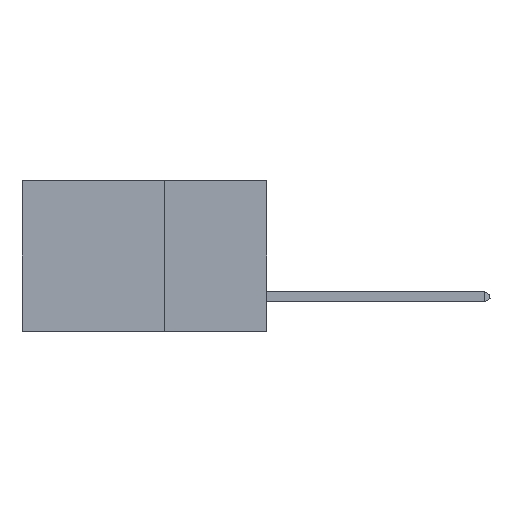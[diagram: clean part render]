
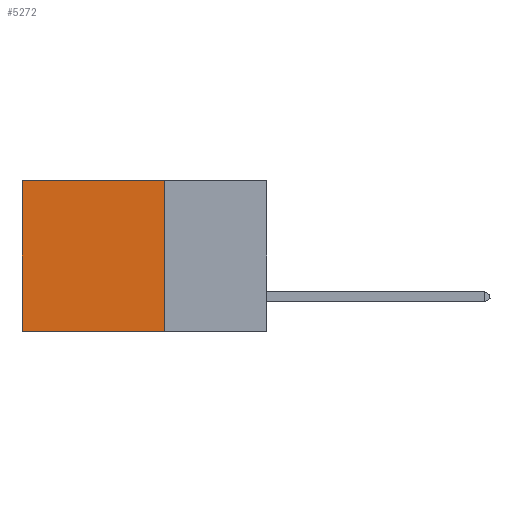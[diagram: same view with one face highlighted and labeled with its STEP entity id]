
A CAD part, left-side view. The second image highlights one B-rep face of the part: STEP entity #5272.
In plain terms, the highlighted planar face has unit normal (-1, 0, 0).
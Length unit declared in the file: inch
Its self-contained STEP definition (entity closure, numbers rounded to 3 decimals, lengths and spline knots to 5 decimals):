
#1403 = CARTESIAN_POINT ( 'NONE',  ( 0.2875, 0.25, -0.37 ) ) ;
#1807 = ORIENTED_EDGE ( 'NONE', *, *, #14989, .T. ) ;
#1818 = VERTEX_POINT ( 'NONE', #23253 ) ;
#1968 = LINE ( 'NONE', #18146, #23484 ) ;
#2635 = DIRECTION ( 'NONE',  ( 0., 0., -1. ) ) ;
#5272 = ADVANCED_FACE ( 'NONE', ( #17365 ), #20144, .F. ) ;
#7368 = CARTESIAN_POINT ( 'NONE',  ( 0.2875, 0.25, -0.37 ) ) ;
#7627 = DIRECTION ( 'NONE',  ( 0., 0., -1. ) ) ;
#8122 = CARTESIAN_POINT ( 'NONE',  ( 0.2875, 0.25, 0. ) ) ;
#8466 = EDGE_LOOP ( 'NONE', ( #1807, #14694, #33051, #15917 ) ) ;
#9896 = CARTESIAN_POINT ( 'NONE',  ( 0.2875, 0.25, 0. ) ) ;
#10427 = LINE ( 'NONE', #16208, #32858 ) ;
#11057 = VERTEX_POINT ( 'NONE', #1403 ) ;
#12004 = DIRECTION ( 'NONE',  ( 0., 1., 0. ) ) ;
#14694 = ORIENTED_EDGE ( 'NONE', *, *, #29916, .F. ) ;
#14989 = EDGE_CURVE ( 'NONE', #27148, #1818, #10427, .T. ) ;
#15917 = ORIENTED_EDGE ( 'NONE', *, *, #20782, .T. ) ;
#16208 = CARTESIAN_POINT ( 'NONE',  ( 0.2875, 0.6, 0. ) ) ;
#17365 = FACE_OUTER_BOUND ( 'NONE', #8466, .T. ) ;
#18146 = CARTESIAN_POINT ( 'NONE',  ( 0.2875, 0.25, 0. ) ) ;
#19039 = VECTOR ( 'NONE', #12004, 39.37008 ) ;
#19268 = DIRECTION ( 'NONE',  ( 0., 1., 0. ) ) ;
#20144 = PLANE ( 'NONE',  #24566 ) ;
#20782 = EDGE_CURVE ( 'NONE', #34213, #27148, #37319, .T. ) ;
#20951 = LINE ( 'NONE', #7368, #28779 ) ;
#23253 = CARTESIAN_POINT ( 'NONE',  ( 0.2875, 0.6, -0.37 ) ) ;
#23484 = VECTOR ( 'NONE', #35566, 39.37008 ) ;
#24070 = EDGE_CURVE ( 'NONE', #34213, #11057, #1968, .T. ) ;
#24566 = AXIS2_PLACEMENT_3D ( 'NONE', #8122, #28987, #2635 ) ;
#27148 = VERTEX_POINT ( 'NONE', #29777 ) ;
#28779 = VECTOR ( 'NONE', #19268, 39.37008 ) ;
#28987 = DIRECTION ( 'NONE',  ( 1., 0., 0. ) ) ;
#29402 = CARTESIAN_POINT ( 'NONE',  ( 0.2875, 0.25, 0. ) ) ;
#29777 = CARTESIAN_POINT ( 'NONE',  ( 0.2875, 0.6, 0. ) ) ;
#29916 = EDGE_CURVE ( 'NONE', #11057, #1818, #20951, .T. ) ;
#32858 = VECTOR ( 'NONE', #7627, 39.37008 ) ;
#33051 = ORIENTED_EDGE ( 'NONE', *, *, #24070, .F. ) ;
#34213 = VERTEX_POINT ( 'NONE', #9896 ) ;
#35566 = DIRECTION ( 'NONE',  ( 0., 0., -1. ) ) ;
#37319 = LINE ( 'NONE', #29402, #19039 ) ;
